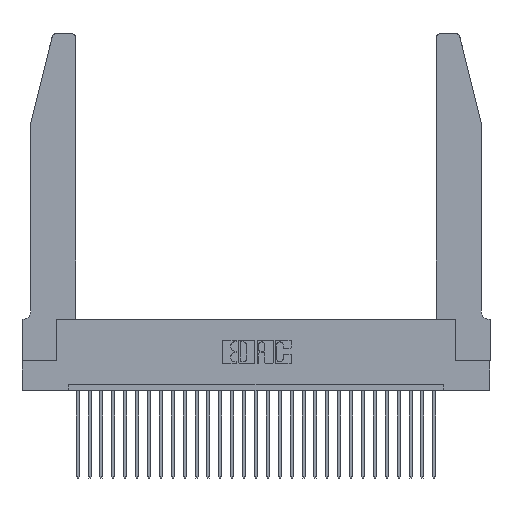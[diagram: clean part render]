
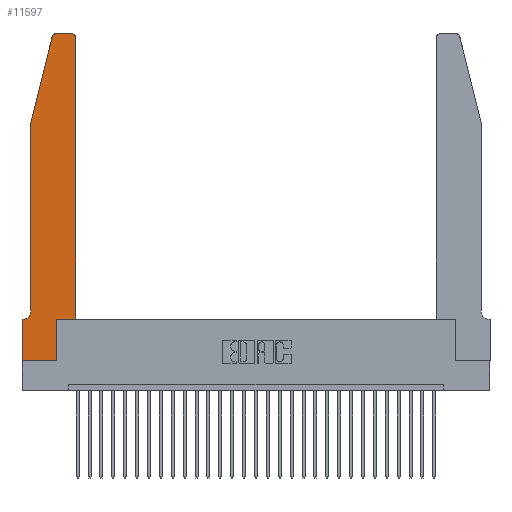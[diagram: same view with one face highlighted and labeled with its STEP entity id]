
A CAD part, top view. The second image highlights one B-rep face of the part: STEP entity #11597.
In plain terms, the highlighted planar face has unit normal (0, 0, 1).
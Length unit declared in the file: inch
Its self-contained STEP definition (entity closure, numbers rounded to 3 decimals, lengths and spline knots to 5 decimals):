
#173 = VECTOR ( 'NONE', #22893, 39.37008 ) ;
#595 = ORIENTED_EDGE ( 'NONE', *, *, #26492, .T. ) ;
#614 = LINE ( 'NONE', #24569, #13179 ) ;
#1139 = CARTESIAN_POINT ( 'NONE',  ( 0.284, 2.75, 0.37 ) ) ;
#1148 = LINE ( 'NONE', #13230, #18641 ) ;
#1215 = VERTEX_POINT ( 'NONE', #17366 ) ;
#1322 = DIRECTION ( 'NONE',  ( 1., 0., 0. ) ) ;
#1499 = FACE_OUTER_BOUND ( 'NONE', #13377, .T. ) ;
#1525 = DIRECTION ( 'NONE',  ( 1., 0., 0. ) ) ;
#1625 = CARTESIAN_POINT ( 'NONE',  ( 0.0755, 0.42, 0.37 ) ) ;
#1669 = ORIENTED_EDGE ( 'NONE', *, *, #23816, .T. ) ;
#1770 = AXIS2_PLACEMENT_3D ( 'NONE', #8138, #17495, #19768 ) ;
#2519 = VECTOR ( 'NONE', #10125, 39.37008 ) ;
#2527 = LINE ( 'NONE', #27892, #8263 ) ;
#3023 = EDGE_CURVE ( 'NONE', #12759, #9393, #4619, .T. ) ;
#3924 = LINE ( 'NONE', #15264, #8567 ) ;
#4162 = VERTEX_POINT ( 'NONE', #9718 ) ;
#4196 = CARTESIAN_POINT ( 'NONE',  ( 0.0755, 2., 0.37 ) ) ;
#4618 = ORIENTED_EDGE ( 'NONE', *, *, #10718, .T. ) ;
#4619 = CIRCLE ( 'NONE', #19970, 0.03 ) ;
#4648 = LINE ( 'NONE', #21658, #2519 ) ;
#5224 = CARTESIAN_POINT ( 'NONE',  ( 0.4505, 2.72, 0.37 ) ) ;
#5699 = LINE ( 'NONE', #4196, #27509 ) ;
#5704 = DIRECTION ( 'NONE',  ( 0., 0., 1. ) ) ;
#5746 = VERTEX_POINT ( 'NONE', #27901 ) ;
#5963 = CARTESIAN_POINT ( 'NONE',  ( 0., 0., 0.37 ) ) ;
#6791 = EDGE_CURVE ( 'NONE', #5746, #24600, #5699, .T. ) ;
#7895 = VERTEX_POINT ( 'NONE', #1139 ) ;
#8138 = CARTESIAN_POINT ( 'NONE',  ( 0.0055, 0.42, 0.37 ) ) ;
#8263 = VECTOR ( 'NONE', #27505, 39.37008 ) ;
#8526 = DIRECTION ( 'NONE',  ( -0.239, -0.971, 0. ) ) ;
#8567 = VECTOR ( 'NONE', #8526, 39.37008 ) ;
#8954 = ORIENTED_EDGE ( 'NONE', *, *, #25878, .T. ) ;
#9393 = VERTEX_POINT ( 'NONE', #15815 ) ;
#9718 = CARTESIAN_POINT ( 'NONE',  ( 0.0055, 0.35, 0.37 ) ) ;
#9848 = DIRECTION ( 'NONE',  ( 1., 0., 0. ) ) ;
#10125 = DIRECTION ( 'NONE',  ( 1., 0., 0. ) ) ;
#10172 = CARTESIAN_POINT ( 'NONE',  ( 0.4205, 2.72, 0.37 ) ) ;
#10207 = CARTESIAN_POINT ( 'NONE',  ( 0.25487, 2.72718, 0.37 ) ) ;
#10259 = PLANE ( 'NONE',  #18203 ) ;
#10521 = EDGE_CURVE ( 'NONE', #4162, #11268, #11816, .T. ) ;
#10718 = EDGE_CURVE ( 'NONE', #12909, #1215, #1148, .T. ) ;
#10776 = CARTESIAN_POINT ( 'NONE',  ( 0.284, 2.72, 0.37 ) ) ;
#11105 = DIRECTION ( 'NONE',  ( 1., 0., 0. ) ) ;
#11268 = VERTEX_POINT ( 'NONE', #22091 ) ;
#11597 = ADVANCED_FACE ( 'NONE', ( #1499 ), #10259, .T. ) ;
#11765 = CARTESIAN_POINT ( 'NONE',  ( 0.2865, 0., 0.37 ) ) ;
#11816 = LINE ( 'NONE', #14678, #19025 ) ;
#12676 = CARTESIAN_POINT ( 'NONE',  ( 0.2865, 0.35, 0.37 ) ) ;
#12759 = VERTEX_POINT ( 'NONE', #5224 ) ;
#12786 = CARTESIAN_POINT ( 'NONE',  ( 0., 0.35, 0.37 ) ) ;
#12909 = VERTEX_POINT ( 'NONE', #12676 ) ;
#12949 = DIRECTION ( 'NONE',  ( 0., -1., 0. ) ) ;
#13066 = ORIENTED_EDGE ( 'NONE', *, *, #3023, .T. ) ;
#13179 = VECTOR ( 'NONE', #19984, 39.37008 ) ;
#13230 = CARTESIAN_POINT ( 'NONE',  ( 0.4505, 0.35, 0.37 ) ) ;
#13377 = EDGE_LOOP ( 'NONE', ( #26129, #595, #28738, #19695, #8954, #20931, #17002, #21465, #1669, #4618, #13677, #13066 ) ) ;
#13390 = DIRECTION ( 'NONE',  ( -1., 0., 0. ) ) ;
#13583 = EDGE_CURVE ( 'NONE', #19755, #5746, #3924, .T. ) ;
#13677 = ORIENTED_EDGE ( 'NONE', *, *, #19006, .T. ) ;
#14678 = CARTESIAN_POINT ( 'NONE',  ( 0.0755, 0.35, 0.37 ) ) ;
#14788 = VECTOR ( 'NONE', #12949, 39.37008 ) ;
#15264 = CARTESIAN_POINT ( 'NONE',  ( 0.0755, 2., 0.37 ) ) ;
#15815 = CARTESIAN_POINT ( 'NONE',  ( 0.4205, 2.75, 0.37 ) ) ;
#17002 = ORIENTED_EDGE ( 'NONE', *, *, #25786, .T. ) ;
#17366 = CARTESIAN_POINT ( 'NONE',  ( 0.4505, 0.35, 0.37 ) ) ;
#17495 = DIRECTION ( 'NONE',  ( 0., 0., -1. ) ) ;
#17948 = EDGE_CURVE ( 'NONE', #9393, #7895, #614, .T. ) ;
#18062 = VERTEX_POINT ( 'NONE', #11765 ) ;
#18203 = AXIS2_PLACEMENT_3D ( 'NONE', #12786, #5704, #1322 ) ;
#18641 = VECTOR ( 'NONE', #11105, 39.37008 ) ;
#19006 = EDGE_CURVE ( 'NONE', #1215, #12759, #23095, .T. ) ;
#19025 = VECTOR ( 'NONE', #13390, 39.37008 ) ;
#19695 = ORIENTED_EDGE ( 'NONE', *, *, #6791, .T. ) ;
#19755 = VERTEX_POINT ( 'NONE', #10207 ) ;
#19768 = DIRECTION ( 'NONE',  ( -1., 0., 0. ) ) ;
#19970 = AXIS2_PLACEMENT_3D ( 'NONE', #10172, #21199, #9848 ) ;
#19984 = DIRECTION ( 'NONE',  ( -1., 0., 0. ) ) ;
#20861 = LINE ( 'NONE', #5963, #14788 ) ;
#20931 = ORIENTED_EDGE ( 'NONE', *, *, #10521, .T. ) ;
#21199 = DIRECTION ( 'NONE',  ( 0., 0., 1. ) ) ;
#21377 = DIRECTION ( 'NONE',  ( 0., -1., 0. ) ) ;
#21465 = ORIENTED_EDGE ( 'NONE', *, *, #27201, .T. ) ;
#21658 = CARTESIAN_POINT ( 'NONE',  ( 0., 0., 0.37 ) ) ;
#22091 = CARTESIAN_POINT ( 'NONE',  ( 0., 0.35, 0.37 ) ) ;
#22893 = DIRECTION ( 'NONE',  ( 0., 1., 0. ) ) ;
#23095 = LINE ( 'NONE', #27103, #173 ) ;
#23740 = CIRCLE ( 'NONE', #1770, 0.07 ) ;
#23816 = EDGE_CURVE ( 'NONE', #18062, #12909, #2527, .T. ) ;
#24102 = CARTESIAN_POINT ( 'NONE',  ( 0., 0., 0.37 ) ) ;
#24569 = CARTESIAN_POINT ( 'NONE',  ( 0.2605, 2.75, 0.37 ) ) ;
#24600 = VERTEX_POINT ( 'NONE', #1625 ) ;
#25004 = VERTEX_POINT ( 'NONE', #24102 ) ;
#25111 = CIRCLE ( 'NONE', #29518, 0.03 ) ;
#25786 = EDGE_CURVE ( 'NONE', #11268, #25004, #20861, .T. ) ;
#25878 = EDGE_CURVE ( 'NONE', #24600, #4162, #23740, .T. ) ;
#26129 = ORIENTED_EDGE ( 'NONE', *, *, #17948, .T. ) ;
#26492 = EDGE_CURVE ( 'NONE', #7895, #19755, #25111, .T. ) ;
#27103 = CARTESIAN_POINT ( 'NONE',  ( 0.4505, 0.35, 0.37 ) ) ;
#27201 = EDGE_CURVE ( 'NONE', #25004, #18062, #4648, .T. ) ;
#27505 = DIRECTION ( 'NONE',  ( 0., 1., 0. ) ) ;
#27509 = VECTOR ( 'NONE', #21377, 39.37008 ) ;
#27892 = CARTESIAN_POINT ( 'NONE',  ( 0.2865, 0.35, 0.37 ) ) ;
#27901 = CARTESIAN_POINT ( 'NONE',  ( 0.0755, 2., 0.37 ) ) ;
#28738 = ORIENTED_EDGE ( 'NONE', *, *, #13583, .T. ) ;
#28867 = DIRECTION ( 'NONE',  ( 0., 0., 1. ) ) ;
#29518 = AXIS2_PLACEMENT_3D ( 'NONE', #10776, #28867, #1525 ) ;
